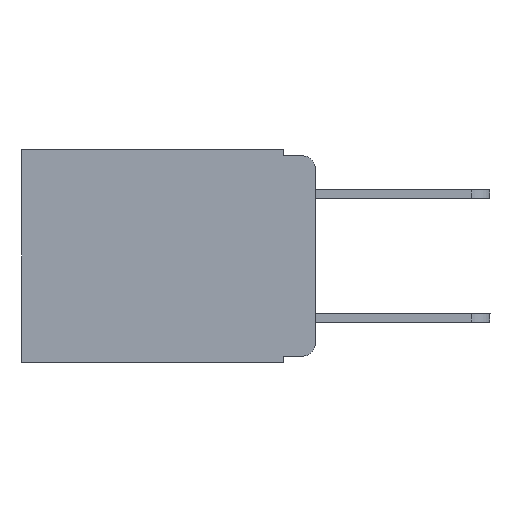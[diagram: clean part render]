
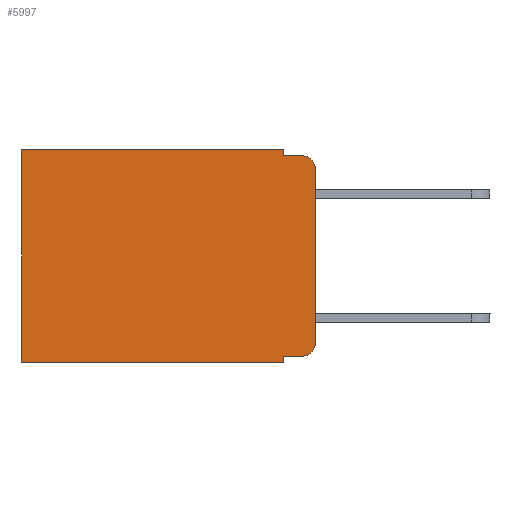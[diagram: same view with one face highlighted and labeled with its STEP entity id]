
A CAD part, left-side view. The second image highlights one B-rep face of the part: STEP entity #5997.
In plain terms, the highlighted planar face has unit normal (-1, 0, 0).
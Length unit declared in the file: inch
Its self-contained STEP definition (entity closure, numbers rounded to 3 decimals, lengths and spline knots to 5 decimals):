
#275 = VERTEX_POINT ( 'NONE', #11522 ) ;
#420 = VERTEX_POINT ( 'NONE', #16372 ) ;
#778 = VECTOR ( 'NONE', #3368, 39.37008 ) ;
#793 = LINE ( 'NONE', #13746, #13855 ) ;
#836 = AXIS2_PLACEMENT_3D ( 'NONE', #3905, #2812, #14043 ) ;
#1234 = ORIENTED_EDGE ( 'NONE', *, *, #9553, .T. ) ;
#1272 = LINE ( 'NONE', #1934, #10950 ) ;
#1574 = DIRECTION ( 'NONE',  ( 0., 0., -1. ) ) ;
#1627 = VERTEX_POINT ( 'NONE', #9353 ) ;
#1788 = DIRECTION ( 'NONE',  ( 1., 0., 0. ) ) ;
#1934 = CARTESIAN_POINT ( 'NONE',  ( 0.298, 0.051, -0.01 ) ) ;
#1985 = ORIENTED_EDGE ( 'NONE', *, *, #6188, .F. ) ;
#2812 = DIRECTION ( 'NONE',  ( -1., 0., 0. ) ) ;
#2958 = EDGE_CURVE ( 'NONE', #420, #275, #793, .T. ) ;
#3163 = EDGE_CURVE ( 'NONE', #6990, #9922, #6124, .T. ) ;
#3368 = DIRECTION ( 'NONE',  ( 0., -1., 0. ) ) ;
#3472 = ORIENTED_EDGE ( 'NONE', *, *, #3163, .T. ) ;
#3576 = CARTESIAN_POINT ( 'NONE',  ( 0.298, 0., -0.03 ) ) ;
#3905 = CARTESIAN_POINT ( 'NONE',  ( 0.298, 0.02, -0.313 ) ) ;
#4130 = EDGE_CURVE ( 'NONE', #7972, #420, #15990, .T. ) ;
#4255 = CARTESIAN_POINT ( 'NONE',  ( 0.298, 0.02, -0.01 ) ) ;
#4271 = VERTEX_POINT ( 'NONE', #4292 ) ;
#4292 = CARTESIAN_POINT ( 'NONE',  ( 0.298, 0.02, -0.333 ) ) ;
#5062 = EDGE_CURVE ( 'NONE', #7972, #4271, #9862, .T. ) ;
#5303 = DIRECTION ( 'NONE',  ( 0., 0., -1. ) ) ;
#5319 = VECTOR ( 'NONE', #15632, 39.37008 ) ;
#5356 = CARTESIAN_POINT ( 'NONE',  ( 0.298, 0.051, 0. ) ) ;
#5540 = LINE ( 'NONE', #11962, #9872 ) ;
#5631 = DIRECTION ( 'NONE',  ( 0., 0., -1. ) ) ;
#5997 = ADVANCED_FACE ( 'NONE', ( #6510 ), #10736, .F. ) ;
#6124 = LINE ( 'NONE', #11826, #5319 ) ;
#6164 = CARTESIAN_POINT ( 'NONE',  ( 0.298, 0.051, -0.333 ) ) ;
#6182 = AXIS2_PLACEMENT_3D ( 'NONE', #14139, #6547, #1574 ) ;
#6188 = EDGE_CURVE ( 'NONE', #11862, #15517, #5540, .T. ) ;
#6226 = EDGE_CURVE ( 'NONE', #9922, #275, #9276, .T. ) ;
#6510 = FACE_OUTER_BOUND ( 'NONE', #12978, .T. ) ;
#6547 = DIRECTION ( 'NONE',  ( -1., 0., 0. ) ) ;
#6633 = ORIENTED_EDGE ( 'NONE', *, *, #5062, .T. ) ;
#6718 = CARTESIAN_POINT ( 'NONE',  ( 0.298, 0., 0. ) ) ;
#6877 = VECTOR ( 'NONE', #10544, 39.37008 ) ;
#6990 = VERTEX_POINT ( 'NONE', #8722 ) ;
#7153 = AXIS2_PLACEMENT_3D ( 'NONE', #6718, #1788, #10625 ) ;
#7972 = VERTEX_POINT ( 'NONE', #6164 ) ;
#8325 = CARTESIAN_POINT ( 'NONE',  ( 0.298, 0.473, 0. ) ) ;
#8604 = CARTESIAN_POINT ( 'NONE',  ( 0.298, 0.051, -0.333 ) ) ;
#8722 = CARTESIAN_POINT ( 'NONE',  ( 0.298, 0.051, 0. ) ) ;
#9015 = EDGE_CURVE ( 'NONE', #6990, #1627, #14931, .T. ) ;
#9173 = EDGE_CURVE ( 'NONE', #1627, #15546, #1272, .T. ) ;
#9276 = LINE ( 'NONE', #8325, #14028 ) ;
#9353 = CARTESIAN_POINT ( 'NONE',  ( 0.298, 0.051, -0.01 ) ) ;
#9391 = DIRECTION ( 'NONE',  ( 0., -1., 0. ) ) ;
#9489 = ORIENTED_EDGE ( 'NONE', *, *, #6226, .T. ) ;
#9553 = EDGE_CURVE ( 'NONE', #4271, #15517, #15900, .T. ) ;
#9575 = VECTOR ( 'NONE', #5303, 39.37008 ) ;
#9862 = LINE ( 'NONE', #8604, #778 ) ;
#9872 = VECTOR ( 'NONE', #5631, 39.37008 ) ;
#9921 = DIRECTION ( 'NONE',  ( 0., 1., 0. ) ) ;
#9922 = VERTEX_POINT ( 'NONE', #12123 ) ;
#10544 = DIRECTION ( 'NONE',  ( 0., 0., -1. ) ) ;
#10625 = DIRECTION ( 'NONE',  ( 0., 0., -1. ) ) ;
#10736 = PLANE ( 'NONE',  #7153 ) ;
#10950 = VECTOR ( 'NONE', #9391, 39.37008 ) ;
#11120 = ORIENTED_EDGE ( 'NONE', *, *, #14376, .T. ) ;
#11202 = ORIENTED_EDGE ( 'NONE', *, *, #4130, .F. ) ;
#11451 = CIRCLE ( 'NONE', #6182, 0.02 ) ;
#11522 = CARTESIAN_POINT ( 'NONE',  ( 0.298, 0.473, -0.343 ) ) ;
#11550 = CARTESIAN_POINT ( 'NONE',  ( 0.298, 0., -0.313 ) ) ;
#11826 = CARTESIAN_POINT ( 'NONE',  ( 0.298, 0., 0. ) ) ;
#11862 = VERTEX_POINT ( 'NONE', #3576 ) ;
#11962 = CARTESIAN_POINT ( 'NONE',  ( 0.298, 0., 0. ) ) ;
#12123 = CARTESIAN_POINT ( 'NONE',  ( 0.298, 0.473, 0. ) ) ;
#12492 = ORIENTED_EDGE ( 'NONE', *, *, #9173, .F. ) ;
#12978 = EDGE_LOOP ( 'NONE', ( #1985, #11120, #12492, #13405, #3472, #9489, #14773, #11202, #6633, #1234 ) ) ;
#12990 = CARTESIAN_POINT ( 'NONE',  ( 0.298, 0.051, 0. ) ) ;
#13405 = ORIENTED_EDGE ( 'NONE', *, *, #9015, .F. ) ;
#13746 = CARTESIAN_POINT ( 'NONE',  ( 0.298, 0., -0.343 ) ) ;
#13855 = VECTOR ( 'NONE', #9921, 39.37008 ) ;
#14028 = VECTOR ( 'NONE', #14595, 39.37008 ) ;
#14043 = DIRECTION ( 'NONE',  ( 0., 0., -1. ) ) ;
#14139 = CARTESIAN_POINT ( 'NONE',  ( 0.298, 0.02, -0.03 ) ) ;
#14376 = EDGE_CURVE ( 'NONE', #11862, #15546, #11451, .T. ) ;
#14595 = DIRECTION ( 'NONE',  ( 0., 0., -1. ) ) ;
#14773 = ORIENTED_EDGE ( 'NONE', *, *, #2958, .F. ) ;
#14931 = LINE ( 'NONE', #12990, #9575 ) ;
#15517 = VERTEX_POINT ( 'NONE', #11550 ) ;
#15546 = VERTEX_POINT ( 'NONE', #4255 ) ;
#15632 = DIRECTION ( 'NONE',  ( 0., 1., 0. ) ) ;
#15900 = CIRCLE ( 'NONE', #836, 0.02 ) ;
#15990 = LINE ( 'NONE', #5356, #6877 ) ;
#16372 = CARTESIAN_POINT ( 'NONE',  ( 0.298, 0.051, -0.343 ) ) ;
